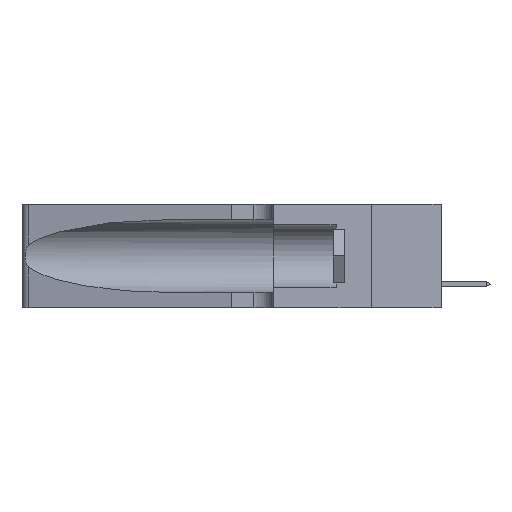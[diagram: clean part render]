
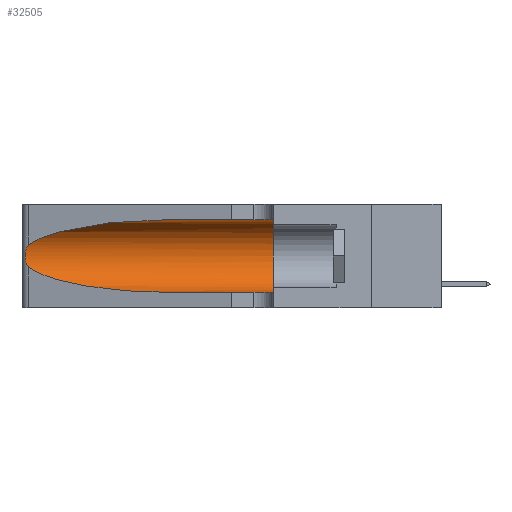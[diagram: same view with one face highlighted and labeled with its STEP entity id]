
A CAD part, left-side view. The second image highlights one B-rep face of the part: STEP entity #32505.
In plain terms, the highlighted cylindrical face has radius 3.308 mm (diameter 6.617 mm), a partial arc.
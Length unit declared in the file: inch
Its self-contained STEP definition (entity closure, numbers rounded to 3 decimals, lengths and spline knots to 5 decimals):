
#557 = CARTESIAN_POINT ( 'NONE',  ( 0.1305, 1.61858, 0.185 ) ) ;
#607 = ORIENTED_EDGE ( 'NONE', *, *, #9285, .F. ) ;
#624 = LINE ( 'NONE', #38100, #39800 ) ;
#2573 = CARTESIAN_POINT ( 'NONE',  ( 0.18966, 0.96281, 0.05475 ) ) ;
#3662 = CYLINDRICAL_SURFACE ( 'NONE', #41980, 0.13025 ) ;
#4130 = CARTESIAN_POINT ( 'NONE',  ( 0.25487, 1.22718, 0.22369 ) ) ;
#4705 = CARTESIAN_POINT ( 'NONE',  ( 0.26018, 1.23835, 0.19895 ) ) ;
#4989 = CARTESIAN_POINT ( 'NONE',  ( 0.1305, 0.35, 0.185 ) ) ;
#5615 = CARTESIAN_POINT ( 'NONE',  ( 0.25487, 1.22718, 0.14631 ) ) ;
#6928 = ORIENTED_EDGE ( 'NONE', *, *, #36675, .T. ) ;
#7627 = CARTESIAN_POINT ( 'NONE',  ( 0.25555, 1.22994, 0.2215 ) ) ;
#7813 = CARTESIAN_POINT ( 'NONE',  ( 0.25487, 1.22718, 0.14631 ) ) ;
#8427 = VERTEX_POINT ( 'NONE', #12571 ) ;
#8678 = DIRECTION ( 'NONE',  ( 0., 1., 0. ) ) ;
#8874 = DIRECTION ( 'NONE',  ( 0., -1., 0. ) ) ;
#9285 = EDGE_CURVE ( 'NONE', #33630, #8427, #40581, .T. ) ;
#9640 = EDGE_CURVE ( 'NONE', #12323, #27386, #27540, .T. ) ;
#9909 = CARTESIAN_POINT ( 'NONE',  ( 0.18966, 0.96281, 0.31525 ) ) ;
#10260 = ORIENTED_EDGE ( 'NONE', *, *, #40905, .T. ) ;
#10524 = EDGE_CURVE ( 'NONE', #11279, #12323, #32190, .T. ) ;
#10569 = DIRECTION ( 'NONE',  ( 0., 0., -1. ) ) ;
#11024 = CARTESIAN_POINT ( 'NONE',  ( 0.26075, 1.23896, 0.19203 ) ) ;
#11173 = CARTESIAN_POINT ( 'NONE',  ( 0.26017, 1.23833, 0.17102 ) ) ;
#11279 = VERTEX_POINT ( 'NONE', #28986 ) ;
#12323 = VERTEX_POINT ( 'NONE', #21226 ) ;
#12567 = CARTESIAN_POINT ( 'NONE',  ( 0.1305, 0.72297, 0.05475 ) ) ;
#12571 = CARTESIAN_POINT ( 'NONE',  ( 0.1305, 0.35, 0.05475 ) ) ;
#13503 =( BOUNDED_CURVE ( )  B_SPLINE_CURVE ( 3, ( #5615, #32779, #2573, #12567 ),
 .UNSPECIFIED., .F., .T. ) 
 B_SPLINE_CURVE_WITH_KNOTS ( ( 4, 4 ),
 ( 3.44316, 4.71239 ),
 .UNSPECIFIED. ) 
 CURVE ( )  GEOMETRIC_REPRESENTATION_ITEM ( )  RATIONAL_B_SPLINE_CURVE ( ( 1., 0.87, 0.87, 1. ) ) 
 REPRESENTATION_ITEM ( '' )  );
#14175 = DIRECTION ( 'NONE',  ( 0., -1., 0. ) ) ;
#14285 = CARTESIAN_POINT ( 'NONE',  ( 0.25787, 1.23484, 0.2124 ) ) ;
#14451 = CARTESIAN_POINT ( 'NONE',  ( 0.25487, 1.22718, 0.14631 ) ) ;
#14888 = CARTESIAN_POINT ( 'NONE',  ( 0.26075, 1.23896, 0.178 ) ) ;
#16086 = DIRECTION ( 'NONE',  ( 0., 0., 1. ) ) ;
#17242 = DIRECTION ( 'NONE',  ( 0., -1., 0. ) ) ;
#17682 = CARTESIAN_POINT ( 'NONE',  ( 0.25854, 1.2359, 0.20912 ) ) ;
#17991 = EDGE_LOOP ( 'NONE', ( #26381, #32359, #6928, #10260, #607, #26524 ) ) ;
#20307 = LINE ( 'NONE', #42776, #27651 ) ;
#21226 = CARTESIAN_POINT ( 'NONE',  ( 0.25487, 1.22718, 0.22369 ) ) ;
#22502 = EDGE_CURVE ( 'NONE', #11279, #33630, #624, .T. ) ;
#23068 = VERTEX_POINT ( 'NONE', #36372 ) ;
#23524 = CARTESIAN_POINT ( 'NONE',  ( 0.25487, 1.22718, 0.22369 ) ) ;
#23941 = AXIS2_PLACEMENT_3D ( 'NONE', #4989, #8678, #16086 ) ;
#24732 = FACE_OUTER_BOUND ( 'NONE', #17991, .T. ) ;
#26381 = ORIENTED_EDGE ( 'NONE', *, *, #10524, .T. ) ;
#26524 = ORIENTED_EDGE ( 'NONE', *, *, #22502, .F. ) ;
#27386 = VERTEX_POINT ( 'NONE', #7813 ) ;
#27540 = B_SPLINE_CURVE_WITH_KNOTS ( 'NONE', 3,
 ( #4130, #7627, #34530, #14285, #17682, #4705, #11024, #14888, #11173, #41186, #34670, #27983, #41618, #14451 ),
 .UNSPECIFIED., .F., .F.,
 ( 4, 2, 2, 2, 2, 2, 4 ),
 ( 0., 0.00027, 0.00053, 0.00107, 0.0016, 0.00187, 0.00214 ),
 .UNSPECIFIED. ) ;
#27651 = VECTOR ( 'NONE', #8874, 39.37008 ) ;
#27983 = CARTESIAN_POINT ( 'NONE',  ( 0.25639, 1.23186, 0.15144 ) ) ;
#28986 = CARTESIAN_POINT ( 'NONE',  ( 0.1305, 0.72297, 0.31525 ) ) ;
#32190 =( BOUNDED_CURVE ( )  B_SPLINE_CURVE ( 3, ( #40634, #9909, #40767, #23524 ),
 .UNSPECIFIED., .F., .F. ) 
 B_SPLINE_CURVE_WITH_KNOTS ( ( 4, 4 ),
 ( 1.5708, 2.84003 ),
 .UNSPECIFIED. ) 
 CURVE ( )  GEOMETRIC_REPRESENTATION_ITEM ( )  RATIONAL_B_SPLINE_CURVE ( ( 1., 0.87, 0.87, 1. ) ) 
 REPRESENTATION_ITEM ( '' )  );
#32359 = ORIENTED_EDGE ( 'NONE', *, *, #9640, .T. ) ;
#32505 = ADVANCED_FACE ( 'NONE', ( #24732 ), #3662, .F. ) ;
#32779 = CARTESIAN_POINT ( 'NONE',  ( 0.2373, 1.15595, 0.08982 ) ) ;
#33630 = VERTEX_POINT ( 'NONE', #42714 ) ;
#34530 = CARTESIAN_POINT ( 'NONE',  ( 0.25639, 1.23184, 0.21858 ) ) ;
#34670 = CARTESIAN_POINT ( 'NONE',  ( 0.25789, 1.23486, 0.15765 ) ) ;
#36372 = CARTESIAN_POINT ( 'NONE',  ( 0.1305, 0.72297, 0.05475 ) ) ;
#36675 = EDGE_CURVE ( 'NONE', #27386, #23068, #13503, .T. ) ;
#38100 = CARTESIAN_POINT ( 'NONE',  ( 0.1305, 1.61858, 0.31525 ) ) ;
#39800 = VECTOR ( 'NONE', #14175, 39.37008 ) ;
#40581 = CIRCLE ( 'NONE', #23941, 0.13025 ) ;
#40634 = CARTESIAN_POINT ( 'NONE',  ( 0.1305, 0.72297, 0.31525 ) ) ;
#40767 = CARTESIAN_POINT ( 'NONE',  ( 0.2373, 1.15595, 0.28018 ) ) ;
#40905 = EDGE_CURVE ( 'NONE', #23068, #8427, #20307, .T. ) ;
#41186 = CARTESIAN_POINT ( 'NONE',  ( 0.25856, 1.23593, 0.16098 ) ) ;
#41618 = CARTESIAN_POINT ( 'NONE',  ( 0.25555, 1.22993, 0.14849 ) ) ;
#41980 = AXIS2_PLACEMENT_3D ( 'NONE', #557, #17242, #10569 ) ;
#42714 = CARTESIAN_POINT ( 'NONE',  ( 0.1305, 0.35, 0.31525 ) ) ;
#42776 = CARTESIAN_POINT ( 'NONE',  ( 0.1305, 1.61858, 0.05475 ) ) ;
